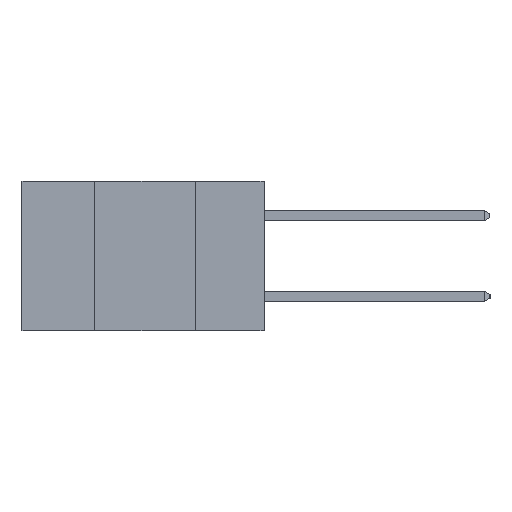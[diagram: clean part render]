
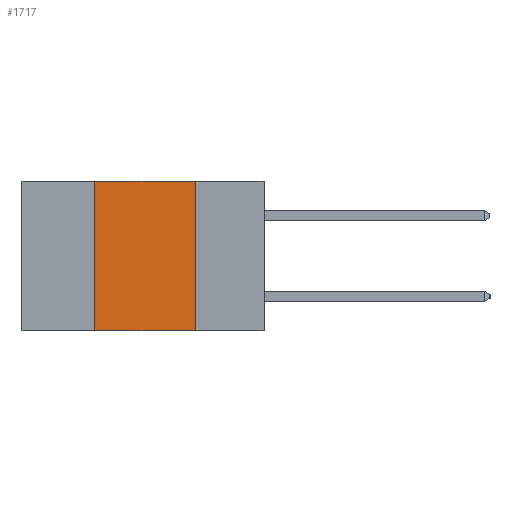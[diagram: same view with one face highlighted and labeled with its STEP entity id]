
A CAD part, left-side view. The second image highlights one B-rep face of the part: STEP entity #1717.
In plain terms, the highlighted planar face has unit normal (-1, 0, 0).
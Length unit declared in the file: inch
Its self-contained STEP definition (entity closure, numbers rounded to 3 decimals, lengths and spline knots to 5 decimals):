
#516 = VERTEX_POINT ( 'NONE', #1652 ) ;
#1374 = CARTESIAN_POINT ( 'NONE',  ( 0., 0.6, -0.37 ) ) ;
#1419 = DIRECTION ( 'NONE',  ( 0., -1., 0. ) ) ;
#1532 = VERTEX_POINT ( 'NONE', #7718 ) ;
#1652 = CARTESIAN_POINT ( 'NONE',  ( 0., 0.42, 0. ) ) ;
#1717 = ADVANCED_FACE ( 'NONE', ( #4610 ), #7958, .F. ) ;
#1720 = VECTOR ( 'NONE', #3451, 39.37008 ) ;
#2109 = ORIENTED_EDGE ( 'NONE', *, *, #4617, .F. ) ;
#2438 = EDGE_CURVE ( 'NONE', #4711, #1532, #5386, .T. ) ;
#3356 = EDGE_CURVE ( 'NONE', #4711, #516, #8029, .T. ) ;
#3373 = CARTESIAN_POINT ( 'NONE',  ( 0., 0.6, 0. ) ) ;
#3451 = DIRECTION ( 'NONE',  ( 0., 0., -1. ) ) ;
#3603 = LINE ( 'NONE', #3373, #8301 ) ;
#4610 = FACE_OUTER_BOUND ( 'NONE', #6549, .T. ) ;
#4617 = EDGE_CURVE ( 'NONE', #516, #5587, #3603, .T. ) ;
#4646 = ORIENTED_EDGE ( 'NONE', *, *, #7236, .F. ) ;
#4686 = CARTESIAN_POINT ( 'NONE',  ( 0., 0.17, 0. ) ) ;
#4711 = VERTEX_POINT ( 'NONE', #6648 ) ;
#5219 = DIRECTION ( 'NONE',  ( 0., 0., -1. ) ) ;
#5330 = AXIS2_PLACEMENT_3D ( 'NONE', #6996, #6141, #5219 ) ;
#5386 = LINE ( 'NONE', #1374, #8659 ) ;
#5474 = ORIENTED_EDGE ( 'NONE', *, *, #2438, .T. ) ;
#5587 = VERTEX_POINT ( 'NONE', #4686 ) ;
#5839 = LINE ( 'NONE', #7317, #1720 ) ;
#6141 = DIRECTION ( 'NONE',  ( 1., 0., 0. ) ) ;
#6307 = VECTOR ( 'NONE', #7732, 39.37008 ) ;
#6549 = EDGE_LOOP ( 'NONE', ( #4646, #2109, #7402, #5474 ) ) ;
#6648 = CARTESIAN_POINT ( 'NONE',  ( 0., 0.42, -0.37 ) ) ;
#6996 = CARTESIAN_POINT ( 'NONE',  ( 0., 0.6, 0. ) ) ;
#7220 = DIRECTION ( 'NONE',  ( 0., -1., 0. ) ) ;
#7236 = EDGE_CURVE ( 'NONE', #5587, #1532, #5839, .T. ) ;
#7317 = CARTESIAN_POINT ( 'NONE',  ( 0., 0.17, -0.37 ) ) ;
#7402 = ORIENTED_EDGE ( 'NONE', *, *, #3356, .F. ) ;
#7718 = CARTESIAN_POINT ( 'NONE',  ( 0., 0.17, -0.37 ) ) ;
#7732 = DIRECTION ( 'NONE',  ( 0., 0., 1. ) ) ;
#7958 = PLANE ( 'NONE',  #5330 ) ;
#8029 = LINE ( 'NONE', #8316, #6307 ) ;
#8301 = VECTOR ( 'NONE', #7220, 39.37008 ) ;
#8316 = CARTESIAN_POINT ( 'NONE',  ( 0., 0.42, -0.37 ) ) ;
#8659 = VECTOR ( 'NONE', #1419, 39.37008 ) ;
